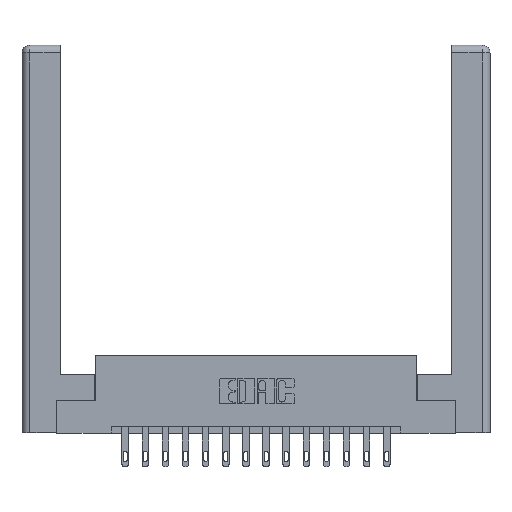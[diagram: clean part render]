
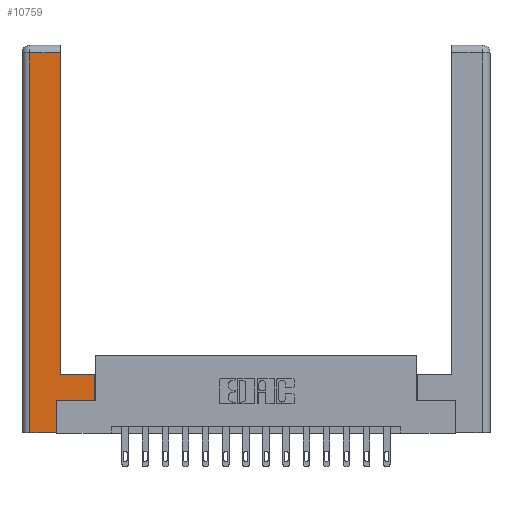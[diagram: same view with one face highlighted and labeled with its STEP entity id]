
A CAD part, top view. The second image highlights one B-rep face of the part: STEP entity #10759.
In plain terms, the highlighted planar face has unit normal (0, 0, 1).
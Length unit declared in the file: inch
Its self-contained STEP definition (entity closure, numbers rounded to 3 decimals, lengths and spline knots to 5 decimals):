
#103 = VECTOR ( 'NONE', #11647, 39.37008 ) ;
#341 = EDGE_CURVE ( 'NONE', #12704, #5584, #2810, .T. ) ;
#353 = CARTESIAN_POINT ( 'NONE',  ( 0.0615, 2.94, 0. ) ) ;
#423 = CARTESIAN_POINT ( 'NONE',  ( 0.265, 0., 0. ) ) ;
#504 = EDGE_CURVE ( 'NONE', #5584, #3250, #11667, .T. ) ;
#571 = DIRECTION ( 'NONE',  ( 0., 0., -1. ) ) ;
#688 = CARTESIAN_POINT ( 'NONE',  ( 0.295, 0.45, 0. ) ) ;
#845 = CARTESIAN_POINT ( 'NONE',  ( 0.265, 0.245, 0. ) ) ;
#1501 = VERTEX_POINT ( 'NONE', #688 ) ;
#1720 = DIRECTION ( 'NONE',  ( 0., 1., 0. ) ) ;
#1951 = VECTOR ( 'NONE', #10946, 39.37008 ) ;
#2810 = LINE ( 'NONE', #423, #1951 ) ;
#2989 = EDGE_CURVE ( 'NONE', #16645, #3027, #13843, .T. ) ;
#3027 = VERTEX_POINT ( 'NONE', #13259 ) ;
#3050 = CARTESIAN_POINT ( 'NONE',  ( 0.565, 0.245, 0. ) ) ;
#3250 = VERTEX_POINT ( 'NONE', #5740 ) ;
#3934 = LINE ( 'NONE', #353, #8630 ) ;
#3975 = EDGE_CURVE ( 'NONE', #16427, #16505, #3934, .T. ) ;
#4486 = ORIENTED_EDGE ( 'NONE', *, *, #504, .T. ) ;
#4534 = CARTESIAN_POINT ( 'NONE',  ( 0.565, 0.45, 0. ) ) ;
#4677 = CARTESIAN_POINT ( 'NONE',  ( 0.565, 0.245, 0. ) ) ;
#5274 = EDGE_LOOP ( 'NONE', ( #15779, #8159, #15394, #11763, #4486, #14770, #7338, #10593 ) ) ;
#5584 = VERTEX_POINT ( 'NONE', #16605 ) ;
#5691 = FACE_OUTER_BOUND ( 'NONE', #5274, .T. ) ;
#5740 = CARTESIAN_POINT ( 'NONE',  ( 0.265, 0.245, 0. ) ) ;
#5746 = DIRECTION ( 'NONE',  ( 1., 0., 0. ) ) ;
#6395 = CARTESIAN_POINT ( 'NONE',  ( 0.295, 0.45, 0. ) ) ;
#6673 = LINE ( 'NONE', #16128, #11393 ) ;
#6785 = DIRECTION ( 'NONE',  ( -1., 0., 0. ) ) ;
#6908 = EDGE_CURVE ( 'NONE', #1501, #16427, #6673, .T. ) ;
#7338 = ORIENTED_EDGE ( 'NONE', *, *, #2989, .T. ) ;
#8117 = VECTOR ( 'NONE', #8682, 39.37008 ) ;
#8159 = ORIENTED_EDGE ( 'NONE', *, *, #3975, .T. ) ;
#8417 = CARTESIAN_POINT ( 'NONE',  ( 0., 0., 0. ) ) ;
#8630 = VECTOR ( 'NONE', #6785, 39.37008 ) ;
#8682 = DIRECTION ( 'NONE',  ( 0., 1., 0. ) ) ;
#8697 = DIRECTION ( 'NONE',  ( -1., 0., 0. ) ) ;
#8790 = LINE ( 'NONE', #3050, #16088 ) ;
#8802 = VECTOR ( 'NONE', #14638, 39.37008 ) ;
#8867 = CARTESIAN_POINT ( 'NONE',  ( 0.0615, 0., 0. ) ) ;
#9816 = EDGE_CURVE ( 'NONE', #16505, #12704, #15027, .T. ) ;
#10248 = CARTESIAN_POINT ( 'NONE',  ( 0.0615, 0., 0. ) ) ;
#10593 = ORIENTED_EDGE ( 'NONE', *, *, #16111, .T. ) ;
#10759 = ADVANCED_FACE ( 'NONE', ( #5691 ), #16364, .F. ) ;
#10946 = DIRECTION ( 'NONE',  ( 1., 0., 0. ) ) ;
#11393 = VECTOR ( 'NONE', #12306, 39.37008 ) ;
#11647 = DIRECTION ( 'NONE',  ( -1., 0., 0. ) ) ;
#11667 = LINE ( 'NONE', #845, #8117 ) ;
#11763 = ORIENTED_EDGE ( 'NONE', *, *, #341, .T. ) ;
#11820 = VECTOR ( 'NONE', #1720, 39.37008 ) ;
#12306 = DIRECTION ( 'NONE',  ( 0., 1., 0. ) ) ;
#12691 = EDGE_CURVE ( 'NONE', #3250, #16645, #8790, .T. ) ;
#12704 = VERTEX_POINT ( 'NONE', #8867 ) ;
#13259 = CARTESIAN_POINT ( 'NONE',  ( 0.565, 0.45, 0. ) ) ;
#13843 = LINE ( 'NONE', #4534, #11820 ) ;
#14151 = CARTESIAN_POINT ( 'NONE',  ( 0.295, 2.94, 0. ) ) ;
#14277 = LINE ( 'NONE', #6395, #103 ) ;
#14638 = DIRECTION ( 'NONE',  ( 0., -1., 0. ) ) ;
#14770 = ORIENTED_EDGE ( 'NONE', *, *, #12691, .T. ) ;
#15027 = LINE ( 'NONE', #10248, #8802 ) ;
#15115 = AXIS2_PLACEMENT_3D ( 'NONE', #8417, #571, #8697 ) ;
#15394 = ORIENTED_EDGE ( 'NONE', *, *, #9816, .T. ) ;
#15779 = ORIENTED_EDGE ( 'NONE', *, *, #6908, .T. ) ;
#16088 = VECTOR ( 'NONE', #5746, 39.37008 ) ;
#16111 = EDGE_CURVE ( 'NONE', #3027, #1501, #14277, .T. ) ;
#16128 = CARTESIAN_POINT ( 'NONE',  ( 0.295, 3., 0. ) ) ;
#16297 = CARTESIAN_POINT ( 'NONE',  ( 0.0615, 2.94, 0. ) ) ;
#16364 = PLANE ( 'NONE',  #15115 ) ;
#16427 = VERTEX_POINT ( 'NONE', #14151 ) ;
#16505 = VERTEX_POINT ( 'NONE', #16297 ) ;
#16605 = CARTESIAN_POINT ( 'NONE',  ( 0.265, 0., 0. ) ) ;
#16645 = VERTEX_POINT ( 'NONE', #4677 ) ;
